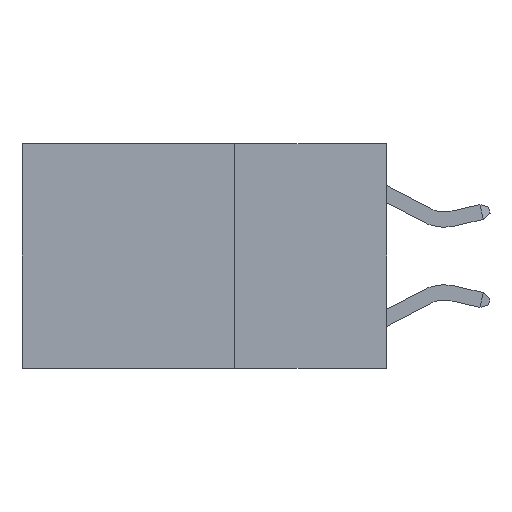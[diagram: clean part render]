
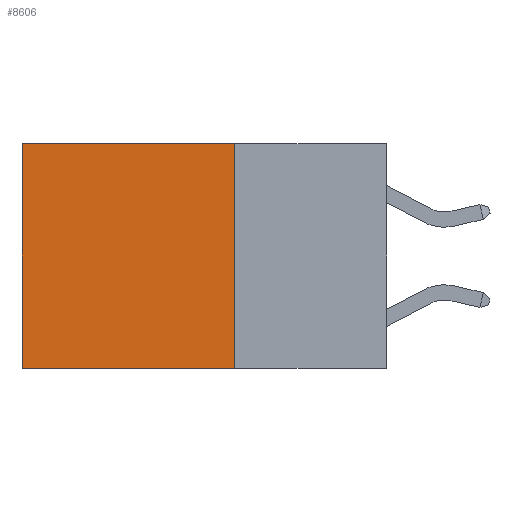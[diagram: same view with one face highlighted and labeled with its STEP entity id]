
A CAD part, left-side view. The second image highlights one B-rep face of the part: STEP entity #8606.
In plain terms, the highlighted planar face has unit normal (-1, 0, 0).
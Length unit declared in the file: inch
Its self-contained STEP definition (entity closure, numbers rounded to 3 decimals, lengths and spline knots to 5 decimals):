
#1120 = DIRECTION ( 'NONE',  ( 0., 1., 0. ) ) ;
#2219 = EDGE_CURVE ( 'NONE', #7736, #13308, #18835, .T. ) ;
#2985 = CARTESIAN_POINT ( 'NONE',  ( 0.2625, 0.6, -0.37 ) ) ;
#3315 = LINE ( 'NONE', #3626, #27908 ) ;
#3581 = DIRECTION ( 'NONE',  ( 0., 0., -1. ) ) ;
#3626 = CARTESIAN_POINT ( 'NONE',  ( 0.2625, 0.6, 0. ) ) ;
#4742 = VERTEX_POINT ( 'NONE', #8084 ) ;
#5614 = DIRECTION ( 'NONE',  ( 0., 0., -1. ) ) ;
#6136 = CARTESIAN_POINT ( 'NONE',  ( 0.2625, 0.25, -0.37 ) ) ;
#6755 = VERTEX_POINT ( 'NONE', #29703 ) ;
#7193 = EDGE_CURVE ( 'NONE', #6755, #4742, #12869, .T. ) ;
#7261 = CARTESIAN_POINT ( 'NONE',  ( 0.2625, 0.25, -0.37 ) ) ;
#7736 = VERTEX_POINT ( 'NONE', #6136 ) ;
#8056 = CARTESIAN_POINT ( 'NONE',  ( 0.2625, 0.25, 0. ) ) ;
#8084 = CARTESIAN_POINT ( 'NONE',  ( 0.2625, 0.6, 0. ) ) ;
#8167 = FACE_OUTER_BOUND ( 'NONE', #29433, .T. ) ;
#8301 = AXIS2_PLACEMENT_3D ( 'NONE', #15144, #24485, #3581 ) ;
#8512 = LINE ( 'NONE', #8056, #20562 ) ;
#8606 = ADVANCED_FACE ( 'NONE', ( #8167 ), #26755, .F. ) ;
#10408 = ORIENTED_EDGE ( 'NONE', *, *, #7193, .T. ) ;
#11929 = ORIENTED_EDGE ( 'NONE', *, *, #17615, .T. ) ;
#12869 = LINE ( 'NONE', #22171, #19905 ) ;
#13308 = VERTEX_POINT ( 'NONE', #2985 ) ;
#15144 = CARTESIAN_POINT ( 'NONE',  ( 0.2625, 0.25, 0. ) ) ;
#17605 = EDGE_CURVE ( 'NONE', #6755, #7736, #8512, .T. ) ;
#17615 = EDGE_CURVE ( 'NONE', #4742, #13308, #3315, .T. ) ;
#18822 = VECTOR ( 'NONE', #23594, 39.37008 ) ;
#18835 = LINE ( 'NONE', #7261, #18822 ) ;
#19610 = DIRECTION ( 'NONE',  ( 0., 0., -1. ) ) ;
#19905 = VECTOR ( 'NONE', #1120, 39.37008 ) ;
#20562 = VECTOR ( 'NONE', #19610, 39.37008 ) ;
#21658 = ORIENTED_EDGE ( 'NONE', *, *, #2219, .F. ) ;
#22171 = CARTESIAN_POINT ( 'NONE',  ( 0.2625, 0.25, 0. ) ) ;
#23594 = DIRECTION ( 'NONE',  ( 0., 1., 0. ) ) ;
#23671 = ORIENTED_EDGE ( 'NONE', *, *, #17605, .F. ) ;
#24485 = DIRECTION ( 'NONE',  ( 1., 0., 0. ) ) ;
#26755 = PLANE ( 'NONE',  #8301 ) ;
#27908 = VECTOR ( 'NONE', #5614, 39.37008 ) ;
#29433 = EDGE_LOOP ( 'NONE', ( #11929, #21658, #23671, #10408 ) ) ;
#29703 = CARTESIAN_POINT ( 'NONE',  ( 0.2625, 0.25, 0. ) ) ;
